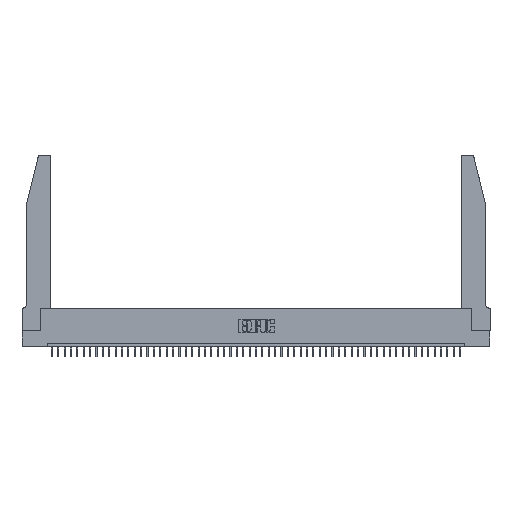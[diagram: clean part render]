
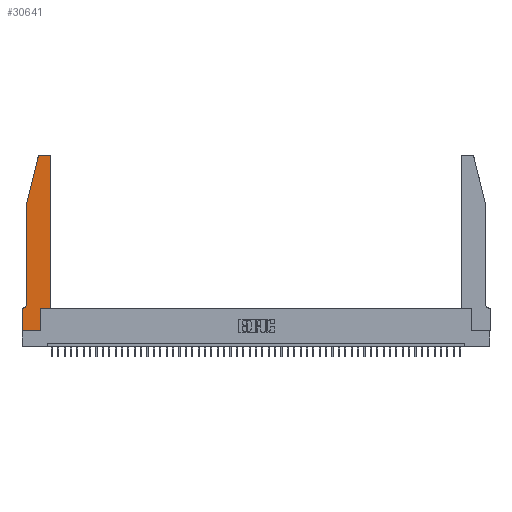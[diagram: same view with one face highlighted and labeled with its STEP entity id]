
A CAD part, top view. The second image highlights one B-rep face of the part: STEP entity #30641.
In plain terms, the highlighted planar face has unit normal (0, 0, 1).
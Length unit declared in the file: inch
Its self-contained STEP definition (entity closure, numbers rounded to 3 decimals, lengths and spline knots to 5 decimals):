
#887 = LINE ( 'NONE', #17466, #19192 ) ;
#1006 = VECTOR ( 'NONE', #1318, 39.37008 ) ;
#1318 = DIRECTION ( 'NONE',  ( 0., 1., 0. ) ) ;
#1482 = LINE ( 'NONE', #22042, #14756 ) ;
#2530 = CARTESIAN_POINT ( 'NONE',  ( 0.4505, 0.35, 0.37 ) ) ;
#2899 = ORIENTED_EDGE ( 'NONE', *, *, #44816, .T. ) ;
#4253 = VERTEX_POINT ( 'NONE', #20606 ) ;
#4414 = CARTESIAN_POINT ( 'NONE',  ( 0.284, 2.72, 0.37 ) ) ;
#4982 = EDGE_CURVE ( 'NONE', #44571, #46555, #13933, .T. ) ;
#5008 = ORIENTED_EDGE ( 'NONE', *, *, #17337, .T. ) ;
#5660 = DIRECTION ( 'NONE',  ( 0., 0., 1. ) ) ;
#5895 = DIRECTION ( 'NONE',  ( -1., 0., 0. ) ) ;
#6739 = CARTESIAN_POINT ( 'NONE',  ( 0.4505, 2.72, 0.37 ) ) ;
#7544 = CARTESIAN_POINT ( 'NONE',  ( 0.0755, 2., 0.37 ) ) ;
#7592 = VECTOR ( 'NONE', #46115, 39.37008 ) ;
#7701 = VERTEX_POINT ( 'NONE', #36923 ) ;
#7744 = ORIENTED_EDGE ( 'NONE', *, *, #27622, .T. ) ;
#9716 = CARTESIAN_POINT ( 'NONE',  ( 0.25487, 2.72718, 0.37 ) ) ;
#11340 = VECTOR ( 'NONE', #46887, 39.37008 ) ;
#11737 = CARTESIAN_POINT ( 'NONE',  ( 0.2865, 0.35, 0.37 ) ) ;
#11841 = ORIENTED_EDGE ( 'NONE', *, *, #46657, .T. ) ;
#12084 = ORIENTED_EDGE ( 'NONE', *, *, #19444, .T. ) ;
#12924 = CARTESIAN_POINT ( 'NONE',  ( 0.2865, 0.35, 0.37 ) ) ;
#13044 = LINE ( 'NONE', #30561, #7592 ) ;
#13147 = EDGE_CURVE ( 'NONE', #32448, #48287, #39530, .T. ) ;
#13275 = VECTOR ( 'NONE', #33674, 39.37008 ) ;
#13521 = DIRECTION ( 'NONE',  ( -1., 0., 0. ) ) ;
#13822 = PLANE ( 'NONE',  #19335 ) ;
#13933 = LINE ( 'NONE', #33506, #13275 ) ;
#14346 = CARTESIAN_POINT ( 'NONE',  ( 0., 0., 0.37 ) ) ;
#14492 = DIRECTION ( 'NONE',  ( 0., 0., 1. ) ) ;
#14756 = VECTOR ( 'NONE', #34036, 39.37008 ) ;
#15061 = ORIENTED_EDGE ( 'NONE', *, *, #4982, .T. ) ;
#15233 = VECTOR ( 'NONE', #24087, 39.37008 ) ;
#16410 = FACE_OUTER_BOUND ( 'NONE', #34640, .T. ) ;
#17218 = CARTESIAN_POINT ( 'NONE',  ( 0.4505, 0.35, 0.37 ) ) ;
#17337 = EDGE_CURVE ( 'NONE', #4253, #7701, #887, .T. ) ;
#17466 = CARTESIAN_POINT ( 'NONE',  ( 0.0755, 0.35, 0.37 ) ) ;
#18465 = EDGE_CURVE ( 'NONE', #20051, #30969, #41162, .T. ) ;
#19192 = VECTOR ( 'NONE', #5895, 39.37008 ) ;
#19335 = AXIS2_PLACEMENT_3D ( 'NONE', #37813, #14492, #38330 ) ;
#19444 = EDGE_CURVE ( 'NONE', #46555, #47174, #31227, .T. ) ;
#19492 = CARTESIAN_POINT ( 'NONE',  ( 0., 0., 0.37 ) ) ;
#20051 = VERTEX_POINT ( 'NONE', #11737 ) ;
#20606 = CARTESIAN_POINT ( 'NONE',  ( 0.0055, 0.35, 0.37 ) ) ;
#20830 = CARTESIAN_POINT ( 'NONE',  ( 0.4205, 2.72, 0.37 ) ) ;
#22042 = CARTESIAN_POINT ( 'NONE',  ( 0., 0., 0.37 ) ) ;
#23571 = LINE ( 'NONE', #19492, #11340 ) ;
#23778 = LINE ( 'NONE', #35583, #15233 ) ;
#23941 = CARTESIAN_POINT ( 'NONE',  ( 0.284, 2.75, 0.37 ) ) ;
#24087 = DIRECTION ( 'NONE',  ( 0., 1., 0. ) ) ;
#24473 = VERTEX_POINT ( 'NONE', #46276 ) ;
#24555 = VECTOR ( 'NONE', #33512, 39.37008 ) ;
#25783 = VERTEX_POINT ( 'NONE', #14346 ) ;
#25834 = CARTESIAN_POINT ( 'NONE',  ( 0.0055, 0.42, 0.37 ) ) ;
#27622 = EDGE_CURVE ( 'NONE', #47174, #32448, #13044, .T. ) ;
#29101 = DIRECTION ( 'NONE',  ( 0., 0., -1. ) ) ;
#30279 = EDGE_CURVE ( 'NONE', #30969, #40445, #23778, .T. ) ;
#30561 = CARTESIAN_POINT ( 'NONE',  ( 0.0755, 2., 0.37 ) ) ;
#30641 = ADVANCED_FACE ( 'NONE', ( #16410 ), #13822, .T. ) ;
#30969 = VERTEX_POINT ( 'NONE', #2530 ) ;
#31227 = CIRCLE ( 'NONE', #35106, 0.03 ) ;
#31597 = DIRECTION ( 'NONE',  ( 0., 0., 1. ) ) ;
#31884 = EDGE_CURVE ( 'NONE', #25783, #24473, #23571, .T. ) ;
#32068 = EDGE_CURVE ( 'NONE', #48287, #4253, #48020, .T. ) ;
#32448 = VERTEX_POINT ( 'NONE', #7544 ) ;
#33506 = CARTESIAN_POINT ( 'NONE',  ( 0.2605, 2.75, 0.37 ) ) ;
#33512 = DIRECTION ( 'NONE',  ( 1., 0., 0. ) ) ;
#33674 = DIRECTION ( 'NONE',  ( -1., 0., 0. ) ) ;
#34036 = DIRECTION ( 'NONE',  ( 0., -1., 0. ) ) ;
#34495 = ORIENTED_EDGE ( 'NONE', *, *, #13147, .T. ) ;
#34640 = EDGE_LOOP ( 'NONE', ( #15061, #12084, #7744, #34495, #39377, #5008, #41443, #36031, #2899, #35614, #45789, #11841 ) ) ;
#35106 = AXIS2_PLACEMENT_3D ( 'NONE', #4414, #31597, #39339 ) ;
#35264 = LINE ( 'NONE', #12924, #1006 ) ;
#35583 = CARTESIAN_POINT ( 'NONE',  ( 0.4505, 0.35, 0.37 ) ) ;
#35614 = ORIENTED_EDGE ( 'NONE', *, *, #18465, .T. ) ;
#36031 = ORIENTED_EDGE ( 'NONE', *, *, #31884, .T. ) ;
#36923 = CARTESIAN_POINT ( 'NONE',  ( 0., 0.35, 0.37 ) ) ;
#37471 = AXIS2_PLACEMENT_3D ( 'NONE', #25834, #29101, #13521 ) ;
#37704 = VECTOR ( 'NONE', #41745, 39.37008 ) ;
#37813 = CARTESIAN_POINT ( 'NONE',  ( 0., 0.35, 0.37 ) ) ;
#38330 = DIRECTION ( 'NONE',  ( 1., 0., 0. ) ) ;
#38356 = CARTESIAN_POINT ( 'NONE',  ( 0.0755, 2., 0.37 ) ) ;
#39339 = DIRECTION ( 'NONE',  ( 1., 0., 0. ) ) ;
#39377 = ORIENTED_EDGE ( 'NONE', *, *, #32068, .T. ) ;
#39530 = LINE ( 'NONE', #38356, #37704 ) ;
#40419 = CARTESIAN_POINT ( 'NONE',  ( 0.0755, 0.42, 0.37 ) ) ;
#40445 = VERTEX_POINT ( 'NONE', #6739 ) ;
#41162 = LINE ( 'NONE', #17218, #24555 ) ;
#41443 = ORIENTED_EDGE ( 'NONE', *, *, #46735, .T. ) ;
#41745 = DIRECTION ( 'NONE',  ( 0., -1., 0. ) ) ;
#42051 = CARTESIAN_POINT ( 'NONE',  ( 0.4205, 2.75, 0.37 ) ) ;
#43024 = AXIS2_PLACEMENT_3D ( 'NONE', #20830, #5660, #48213 ) ;
#44571 = VERTEX_POINT ( 'NONE', #42051 ) ;
#44816 = EDGE_CURVE ( 'NONE', #24473, #20051, #35264, .T. ) ;
#45789 = ORIENTED_EDGE ( 'NONE', *, *, #30279, .T. ) ;
#46115 = DIRECTION ( 'NONE',  ( -0.239, -0.971, 0. ) ) ;
#46276 = CARTESIAN_POINT ( 'NONE',  ( 0.2865, 0., 0.37 ) ) ;
#46555 = VERTEX_POINT ( 'NONE', #23941 ) ;
#46657 = EDGE_CURVE ( 'NONE', #40445, #44571, #47105, .T. ) ;
#46735 = EDGE_CURVE ( 'NONE', #7701, #25783, #1482, .T. ) ;
#46887 = DIRECTION ( 'NONE',  ( 1., 0., 0. ) ) ;
#47105 = CIRCLE ( 'NONE', #43024, 0.03 ) ;
#47174 = VERTEX_POINT ( 'NONE', #9716 ) ;
#48020 = CIRCLE ( 'NONE', #37471, 0.07 ) ;
#48213 = DIRECTION ( 'NONE',  ( 1., 0., 0. ) ) ;
#48287 = VERTEX_POINT ( 'NONE', #40419 ) ;
